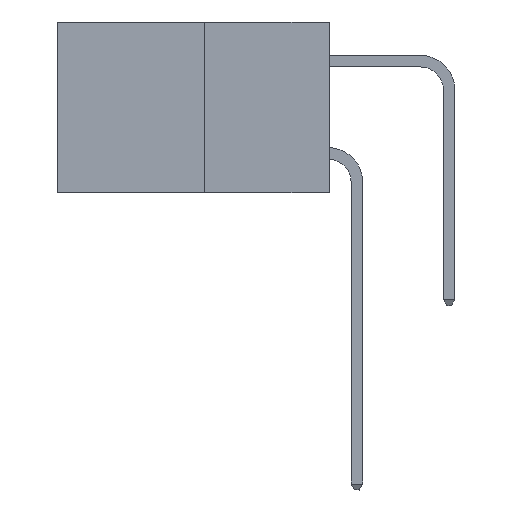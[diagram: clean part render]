
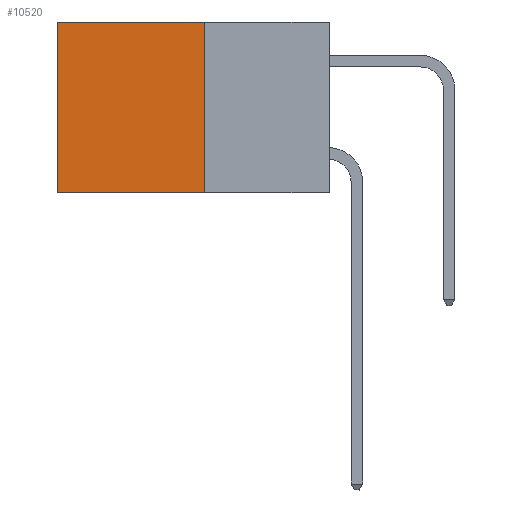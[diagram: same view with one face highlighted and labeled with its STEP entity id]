
A CAD part, left-side view. The second image highlights one B-rep face of the part: STEP entity #10520.
In plain terms, the highlighted planar face has unit normal (-1, 0, 0).
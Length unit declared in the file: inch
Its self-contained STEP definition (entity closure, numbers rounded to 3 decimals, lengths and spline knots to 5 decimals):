
#156 = VERTEX_POINT ( 'NONE', #4141 ) ;
#1126 = EDGE_CURVE ( 'NONE', #1615, #10654, #11661, .T. ) ;
#1265 = EDGE_CURVE ( 'NONE', #156, #1615, #8623, .T. ) ;
#1305 = EDGE_LOOP ( 'NONE', ( #9734, #7106, #4087, #4469 ) ) ;
#1538 = DIRECTION ( 'NONE',  ( 0., 0., -1. ) ) ;
#1615 = VERTEX_POINT ( 'NONE', #2935 ) ;
#1658 = VECTOR ( 'NONE', #3991, 39.37008 ) ;
#2000 = EDGE_CURVE ( 'NONE', #7823, #10654, #9268, .T. ) ;
#2179 = CARTESIAN_POINT ( 'NONE',  ( 0.277, 0.27, -0.37 ) ) ;
#2379 = CARTESIAN_POINT ( 'NONE',  ( 0.277, 0.59, -0.37 ) ) ;
#2935 = CARTESIAN_POINT ( 'NONE',  ( 0.277, 0.27, -0.37 ) ) ;
#3889 = CARTESIAN_POINT ( 'NONE',  ( 0.277, 0.59, 0. ) ) ;
#3991 = DIRECTION ( 'NONE',  ( 0., 1., 0. ) ) ;
#4087 = ORIENTED_EDGE ( 'NONE', *, *, #1265, .F. ) ;
#4141 = CARTESIAN_POINT ( 'NONE',  ( 0.277, 0.27, 0. ) ) ;
#4469 = ORIENTED_EDGE ( 'NONE', *, *, #13824, .T. ) ;
#6086 = CARTESIAN_POINT ( 'NONE',  ( 0.277, 0.27, -0.37 ) ) ;
#6729 = CARTESIAN_POINT ( 'NONE',  ( 0.277, 0.59, -0.37 ) ) ;
#6863 = DIRECTION ( 'NONE',  ( 0., 0., -1. ) ) ;
#6972 = CARTESIAN_POINT ( 'NONE',  ( 0.277, 0.27, -0.37 ) ) ;
#7106 = ORIENTED_EDGE ( 'NONE', *, *, #1126, .F. ) ;
#7823 = VERTEX_POINT ( 'NONE', #3889 ) ;
#7831 = LINE ( 'NONE', #9611, #1658 ) ;
#8623 = LINE ( 'NONE', #6972, #14104 ) ;
#8951 = VECTOR ( 'NONE', #10897, 39.37008 ) ;
#9268 = LINE ( 'NONE', #6729, #8951 ) ;
#9611 = CARTESIAN_POINT ( 'NONE',  ( 0.277, 0.27, 0. ) ) ;
#9734 = ORIENTED_EDGE ( 'NONE', *, *, #2000, .T. ) ;
#10031 = FACE_OUTER_BOUND ( 'NONE', #1305, .T. ) ;
#10520 = ADVANCED_FACE ( 'NONE', ( #10031 ), #12369, .F. ) ;
#10654 = VERTEX_POINT ( 'NONE', #2379 ) ;
#10897 = DIRECTION ( 'NONE',  ( 0., 0., -1. ) ) ;
#11661 = LINE ( 'NONE', #6086, #12396 ) ;
#12369 = PLANE ( 'NONE',  #13704 ) ;
#12396 = VECTOR ( 'NONE', #13513, 39.37008 ) ;
#13494 = DIRECTION ( 'NONE',  ( 1., 0., 0. ) ) ;
#13513 = DIRECTION ( 'NONE',  ( 0., 1., 0. ) ) ;
#13704 = AXIS2_PLACEMENT_3D ( 'NONE', #2179, #13494, #6863 ) ;
#13824 = EDGE_CURVE ( 'NONE', #156, #7823, #7831, .T. ) ;
#14104 = VECTOR ( 'NONE', #1538, 39.37008 ) ;
